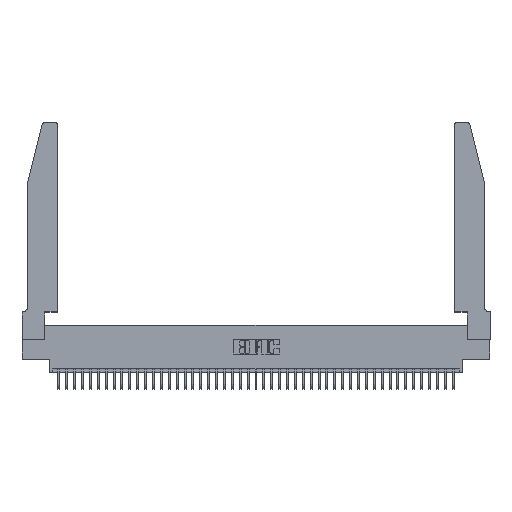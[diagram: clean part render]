
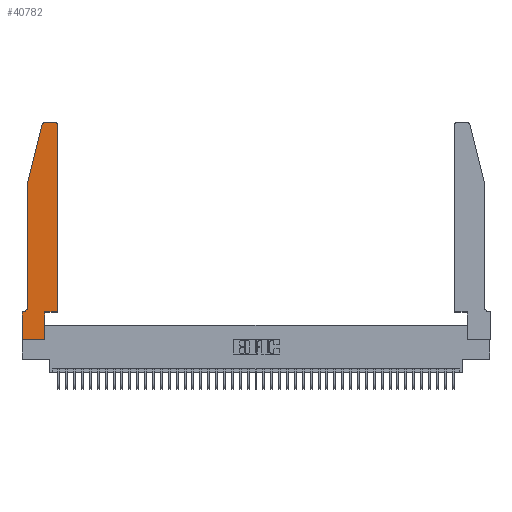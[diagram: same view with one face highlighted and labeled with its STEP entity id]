
A CAD part, top view. The second image highlights one B-rep face of the part: STEP entity #40782.
In plain terms, the highlighted planar face has unit normal (0, 0, 1).
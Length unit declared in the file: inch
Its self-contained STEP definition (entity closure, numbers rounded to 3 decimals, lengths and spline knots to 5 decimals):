
#225 = LINE ( 'NONE', #10814, #11200 ) ;
#509 = DIRECTION ( 'NONE',  ( 0., -1., 0. ) ) ;
#960 = VECTOR ( 'NONE', #30849, 39.37008 ) ;
#1956 = LINE ( 'NONE', #31915, #20055 ) ;
#2452 = CARTESIAN_POINT ( 'NONE',  ( 0.0055, 0.35, 0.37 ) ) ;
#2562 = ORIENTED_EDGE ( 'NONE', *, *, #5323, .T. ) ;
#2713 = LINE ( 'NONE', #25769, #18028 ) ;
#2930 = DIRECTION ( 'NONE',  ( -1., 0., 0. ) ) ;
#3002 = AXIS2_PLACEMENT_3D ( 'NONE', #25650, #27465, #43901 ) ;
#3259 = EDGE_CURVE ( 'NONE', #36909, #41805, #5461, .T. ) ;
#3584 = EDGE_CURVE ( 'NONE', #23288, #6367, #33390, .T. ) ;
#3905 = CARTESIAN_POINT ( 'NONE',  ( 0.25487, 2.72718, 0.37 ) ) ;
#5311 = EDGE_CURVE ( 'NONE', #29956, #12798, #28786, .T. ) ;
#5323 = EDGE_CURVE ( 'NONE', #41805, #23288, #1956, .T. ) ;
#5461 = LINE ( 'NONE', #30258, #21874 ) ;
#6141 = ORIENTED_EDGE ( 'NONE', *, *, #16983, .T. ) ;
#6367 = VERTEX_POINT ( 'NONE', #45171 ) ;
#6553 = ORIENTED_EDGE ( 'NONE', *, *, #5311, .T. ) ;
#6580 = CARTESIAN_POINT ( 'NONE',  ( 0.284, 2.75, 0.37 ) ) ;
#6617 = FACE_OUTER_BOUND ( 'NONE', #28249, .T. ) ;
#7538 = CARTESIAN_POINT ( 'NONE',  ( 0., 0.35, 0.37 ) ) ;
#7981 = ORIENTED_EDGE ( 'NONE', *, *, #24552, .T. ) ;
#8738 = CIRCLE ( 'NONE', #3002, 0.03 ) ;
#8845 = ORIENTED_EDGE ( 'NONE', *, *, #36038, .T. ) ;
#9128 = CARTESIAN_POINT ( 'NONE',  ( 0.4505, 2.72, 0.37 ) ) ;
#10814 = CARTESIAN_POINT ( 'NONE',  ( 0.4505, 0.35, 0.37 ) ) ;
#11200 = VECTOR ( 'NONE', #41607, 39.37008 ) ;
#11848 = CARTESIAN_POINT ( 'NONE',  ( 0., 0., 0.37 ) ) ;
#11878 = DIRECTION ( 'NONE',  ( 0., 0., -1. ) ) ;
#12225 = VERTEX_POINT ( 'NONE', #14831 ) ;
#12562 = VECTOR ( 'NONE', #44334, 39.37008 ) ;
#12609 = ORIENTED_EDGE ( 'NONE', *, *, #18208, .T. ) ;
#12798 = VERTEX_POINT ( 'NONE', #33917 ) ;
#13674 = ORIENTED_EDGE ( 'NONE', *, *, #3259, .T. ) ;
#14398 = VERTEX_POINT ( 'NONE', #6580 ) ;
#14683 = AXIS2_PLACEMENT_3D ( 'NONE', #25961, #11878, #36240 ) ;
#14792 = VERTEX_POINT ( 'NONE', #19567 ) ;
#14831 = CARTESIAN_POINT ( 'NONE',  ( 0.0755, 0.42, 0.37 ) ) ;
#15034 = CARTESIAN_POINT ( 'NONE',  ( 0.2865, 0.35, 0.37 ) ) ;
#15566 = DIRECTION ( 'NONE',  ( 1., 0., 0. ) ) ;
#16915 = EDGE_CURVE ( 'NONE', #12798, #12225, #34268, .T. ) ;
#16983 = EDGE_CURVE ( 'NONE', #12225, #34886, #37588, .T. ) ;
#17345 = CARTESIAN_POINT ( 'NONE',  ( 0.2605, 2.75, 0.37 ) ) ;
#18028 = VECTOR ( 'NONE', #509, 39.37008 ) ;
#18208 = EDGE_CURVE ( 'NONE', #14792, #14398, #19957, .T. ) ;
#18661 = CARTESIAN_POINT ( 'NONE',  ( 0.2865, 0., 0.37 ) ) ;
#19567 = CARTESIAN_POINT ( 'NONE',  ( 0.4205, 2.75, 0.37 ) ) ;
#19957 = LINE ( 'NONE', #17345, #29840 ) ;
#20055 = VECTOR ( 'NONE', #35433, 39.37008 ) ;
#20260 = VERTEX_POINT ( 'NONE', #9128 ) ;
#20475 = ORIENTED_EDGE ( 'NONE', *, *, #16915, .T. ) ;
#20575 = EDGE_CURVE ( 'NONE', #27451, #36909, #2713, .T. ) ;
#20610 = EDGE_CURVE ( 'NONE', #20260, #14792, #8738, .T. ) ;
#20685 = LINE ( 'NONE', #27148, #960 ) ;
#21874 = VECTOR ( 'NONE', #36998, 39.37008 ) ;
#22241 = VECTOR ( 'NONE', #35911, 39.37008 ) ;
#23133 = ORIENTED_EDGE ( 'NONE', *, *, #20575, .T. ) ;
#23222 = CARTESIAN_POINT ( 'NONE',  ( 0., 0.35, 0.37 ) ) ;
#23288 = VERTEX_POINT ( 'NONE', #15034 ) ;
#23778 = CARTESIAN_POINT ( 'NONE',  ( 0.4505, 0.35, 0.37 ) ) ;
#24552 = EDGE_CURVE ( 'NONE', #6367, #20260, #225, .T. ) ;
#25262 = AXIS2_PLACEMENT_3D ( 'NONE', #23222, #36567, #15566 ) ;
#25650 = CARTESIAN_POINT ( 'NONE',  ( 0.4205, 2.72, 0.37 ) ) ;
#25769 = CARTESIAN_POINT ( 'NONE',  ( 0., 0., 0.37 ) ) ;
#25961 = CARTESIAN_POINT ( 'NONE',  ( 0.0055, 0.42, 0.37 ) ) ;
#26402 = ORIENTED_EDGE ( 'NONE', *, *, #20610, .T. ) ;
#26558 = CARTESIAN_POINT ( 'NONE',  ( 0.0755, 2., 0.37 ) ) ;
#26655 = AXIS2_PLACEMENT_3D ( 'NONE', #30546, #29949, #30396 ) ;
#27148 = CARTESIAN_POINT ( 'NONE',  ( 0.0755, 0.35, 0.37 ) ) ;
#27451 = VERTEX_POINT ( 'NONE', #7538 ) ;
#27465 = DIRECTION ( 'NONE',  ( 0., 0., 1. ) ) ;
#27776 = ORIENTED_EDGE ( 'NONE', *, *, #3584, .T. ) ;
#28249 = EDGE_LOOP ( 'NONE', ( #12609, #8845, #6553, #20475, #6141, #36592, #23133, #13674, #2562, #27776, #7981, #26402 ) ) ;
#28786 = LINE ( 'NONE', #26558, #38679 ) ;
#29840 = VECTOR ( 'NONE', #2930, 39.37008 ) ;
#29949 = DIRECTION ( 'NONE',  ( 0., 0., 1. ) ) ;
#29956 = VERTEX_POINT ( 'NONE', #3905 ) ;
#30258 = CARTESIAN_POINT ( 'NONE',  ( 0., 0., 0.37 ) ) ;
#30396 = DIRECTION ( 'NONE',  ( 1., 0., 0. ) ) ;
#30546 = CARTESIAN_POINT ( 'NONE',  ( 0.284, 2.72, 0.37 ) ) ;
#30849 = DIRECTION ( 'NONE',  ( -1., 0., 0. ) ) ;
#31915 = CARTESIAN_POINT ( 'NONE',  ( 0.2865, 0.35, 0.37 ) ) ;
#32312 = CIRCLE ( 'NONE', #26655, 0.03 ) ;
#33390 = LINE ( 'NONE', #23778, #12562 ) ;
#33442 = EDGE_CURVE ( 'NONE', #34886, #27451, #20685, .T. ) ;
#33917 = CARTESIAN_POINT ( 'NONE',  ( 0.0755, 2., 0.37 ) ) ;
#34268 = LINE ( 'NONE', #42447, #22241 ) ;
#34886 = VERTEX_POINT ( 'NONE', #2452 ) ;
#35433 = DIRECTION ( 'NONE',  ( 0., 1., 0. ) ) ;
#35911 = DIRECTION ( 'NONE',  ( 0., -1., 0. ) ) ;
#36038 = EDGE_CURVE ( 'NONE', #14398, #29956, #32312, .T. ) ;
#36240 = DIRECTION ( 'NONE',  ( -1., 0., 0. ) ) ;
#36567 = DIRECTION ( 'NONE',  ( 0., 0., 1. ) ) ;
#36592 = ORIENTED_EDGE ( 'NONE', *, *, #33442, .T. ) ;
#36909 = VERTEX_POINT ( 'NONE', #11848 ) ;
#36998 = DIRECTION ( 'NONE',  ( 1., 0., 0. ) ) ;
#37448 = DIRECTION ( 'NONE',  ( -0.239, -0.971, 0. ) ) ;
#37588 = CIRCLE ( 'NONE', #14683, 0.07 ) ;
#38679 = VECTOR ( 'NONE', #37448, 39.37008 ) ;
#40782 = ADVANCED_FACE ( 'NONE', ( #6617 ), #44208, .T. ) ;
#41607 = DIRECTION ( 'NONE',  ( 0., 1., 0. ) ) ;
#41805 = VERTEX_POINT ( 'NONE', #18661 ) ;
#42447 = CARTESIAN_POINT ( 'NONE',  ( 0.0755, 2., 0.37 ) ) ;
#43901 = DIRECTION ( 'NONE',  ( 1., 0., 0. ) ) ;
#44208 = PLANE ( 'NONE',  #25262 ) ;
#44334 = DIRECTION ( 'NONE',  ( 1., 0., 0. ) ) ;
#45171 = CARTESIAN_POINT ( 'NONE',  ( 0.4505, 0.35, 0.37 ) ) ;
